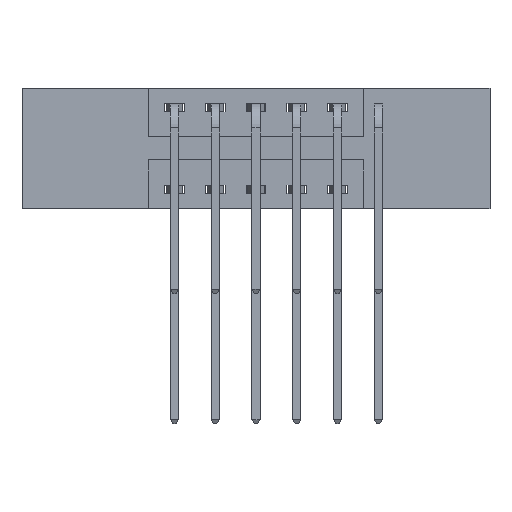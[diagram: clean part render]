
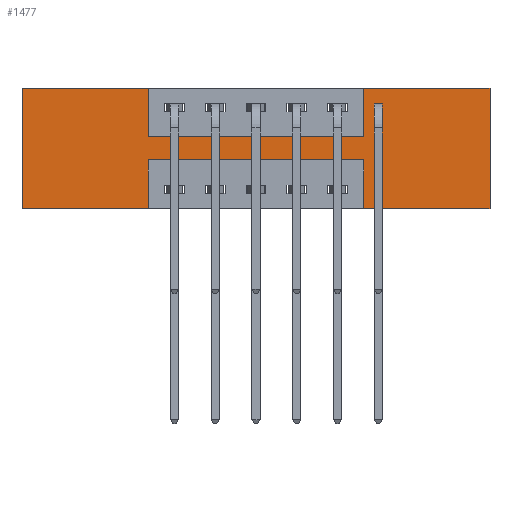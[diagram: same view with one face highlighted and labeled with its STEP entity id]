
A CAD part, front view. The second image highlights one B-rep face of the part: STEP entity #1477.
In plain terms, the highlighted planar face has unit normal (0, -1, 0).
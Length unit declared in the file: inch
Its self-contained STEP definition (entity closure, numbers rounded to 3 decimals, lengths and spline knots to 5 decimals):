
#90 = VERTEX_POINT ( 'NONE', #6516 ) ;
#178 = VERTEX_POINT ( 'NONE', #4496 ) ;
#186 = LINE ( 'NONE', #3003, #9487 ) ;
#317 = CARTESIAN_POINT ( 'NONE',  ( 1.0475, 0., -0.37 ) ) ;
#524 = ORIENTED_EDGE ( 'NONE', *, *, #1689, .F. ) ;
#607 = CARTESIAN_POINT ( 'NONE',  ( 0.3875, 0., 0. ) ) ;
#705 = VECTOR ( 'NONE', #9304, 39.37008 ) ;
#775 = LINE ( 'NONE', #5518, #5379 ) ;
#806 = DIRECTION ( 'NONE',  ( -1., 0., 0. ) ) ;
#931 = LINE ( 'NONE', #4889, #1242 ) ;
#1242 = VECTOR ( 'NONE', #5710, 39.37008 ) ;
#1294 = ORIENTED_EDGE ( 'NONE', *, *, #9307, .F. ) ;
#1436 = CARTESIAN_POINT ( 'NONE',  ( 0., 0., -0.37 ) ) ;
#1477 = ADVANCED_FACE ( 'NONE', ( #8497 ), #6266, .T. ) ;
#1542 = CARTESIAN_POINT ( 'NONE',  ( 1.435, 0., -0.37 ) ) ;
#1647 = DIRECTION ( 'NONE',  ( 0., -1., 0. ) ) ;
#1651 = DIRECTION ( 'NONE',  ( 0., 0., -1. ) ) ;
#1689 = EDGE_CURVE ( 'NONE', #90, #5949, #186, .T. ) ;
#1705 = ORIENTED_EDGE ( 'NONE', *, *, #2231, .F. ) ;
#1850 = EDGE_CURVE ( 'NONE', #178, #90, #4923, .T. ) ;
#2017 = VECTOR ( 'NONE', #806, 39.37008 ) ;
#2084 = VERTEX_POINT ( 'NONE', #607 ) ;
#2087 = ORIENTED_EDGE ( 'NONE', *, *, #7349, .F. ) ;
#2113 = EDGE_CURVE ( 'NONE', #6617, #7820, #9312, .T. ) ;
#2231 = EDGE_CURVE ( 'NONE', #5783, #5242, #9439, .T. ) ;
#2250 = DIRECTION ( 'NONE',  ( 0., 0., 1. ) ) ;
#2278 = DIRECTION ( 'NONE',  ( 1., 0., 0. ) ) ;
#2329 = CARTESIAN_POINT ( 'NONE',  ( 1.0475, 0., -0.22 ) ) ;
#2339 = LINE ( 'NONE', #8656, #8090 ) ;
#2481 = EDGE_CURVE ( 'NONE', #9753, #5783, #4009, .T. ) ;
#2495 = VECTOR ( 'NONE', #9743, 39.37008 ) ;
#2648 = LINE ( 'NONE', #8261, #2495 ) ;
#2877 = EDGE_LOOP ( 'NONE', ( #9728, #7736, #1705, #7483, #2087, #4880, #4223, #6678, #1294, #5826, #524, #3716 ) ) ;
#3003 = CARTESIAN_POINT ( 'NONE',  ( 0., 0., 0. ) ) ;
#3010 = EDGE_CURVE ( 'NONE', #7820, #6430, #2648, .T. ) ;
#3288 = AXIS2_PLACEMENT_3D ( 'NONE', #9418, #1647, #6869 ) ;
#3716 = ORIENTED_EDGE ( 'NONE', *, *, #1850, .F. ) ;
#3961 = VECTOR ( 'NONE', #6442, 39.37008 ) ;
#4009 = LINE ( 'NONE', #1436, #2017 ) ;
#4154 = VERTEX_POINT ( 'NONE', #6844 ) ;
#4171 = CARTESIAN_POINT ( 'NONE',  ( 0.3875, 0., -0.15 ) ) ;
#4223 = ORIENTED_EDGE ( 'NONE', *, *, #3010, .F. ) ;
#4496 = CARTESIAN_POINT ( 'NONE',  ( 0.3875, 0., -0.37 ) ) ;
#4744 = EDGE_CURVE ( 'NONE', #6430, #6102, #775, .T. ) ;
#4880 = ORIENTED_EDGE ( 'NONE', *, *, #4744, .F. ) ;
#4889 = CARTESIAN_POINT ( 'NONE',  ( 0.3875, 0., -0.37 ) ) ;
#4898 = DIRECTION ( 'NONE',  ( 1., 0., 0. ) ) ;
#4923 = LINE ( 'NONE', #6559, #8846 ) ;
#5032 = EDGE_CURVE ( 'NONE', #5949, #2084, #9067, .T. ) ;
#5114 = VECTOR ( 'NONE', #2278, 39.37008 ) ;
#5126 = VECTOR ( 'NONE', #10010, 39.37008 ) ;
#5242 = VERTEX_POINT ( 'NONE', #2329 ) ;
#5379 = VECTOR ( 'NONE', #4898, 39.37008 ) ;
#5499 = CARTESIAN_POINT ( 'NONE',  ( 1.0475, 0., -0.15 ) ) ;
#5518 = CARTESIAN_POINT ( 'NONE',  ( 0., 0., 0. ) ) ;
#5710 = DIRECTION ( 'NONE',  ( 0., 0., -1. ) ) ;
#5783 = VERTEX_POINT ( 'NONE', #317 ) ;
#5826 = ORIENTED_EDGE ( 'NONE', *, *, #5032, .F. ) ;
#5849 = DIRECTION ( 'NONE',  ( -1., 0., 0. ) ) ;
#5949 = VERTEX_POINT ( 'NONE', #8777 ) ;
#6102 = VERTEX_POINT ( 'NONE', #9581 ) ;
#6266 = PLANE ( 'NONE',  #3288 ) ;
#6278 = LINE ( 'NONE', #9433, #8589 ) ;
#6430 = VERTEX_POINT ( 'NONE', #6471 ) ;
#6442 = DIRECTION ( 'NONE',  ( 0., 0., 1. ) ) ;
#6471 = CARTESIAN_POINT ( 'NONE',  ( 1.0475, 0., 0. ) ) ;
#6516 = CARTESIAN_POINT ( 'NONE',  ( 0., 0., -0.37 ) ) ;
#6559 = CARTESIAN_POINT ( 'NONE',  ( 0., 0., -0.37 ) ) ;
#6617 = VERTEX_POINT ( 'NONE', #4171 ) ;
#6678 = ORIENTED_EDGE ( 'NONE', *, *, #2113, .F. ) ;
#6844 = CARTESIAN_POINT ( 'NONE',  ( 0.3875, 0., -0.22 ) ) ;
#6869 = DIRECTION ( 'NONE',  ( 0., 0., -1. ) ) ;
#6899 = LINE ( 'NONE', #8376, #705 ) ;
#6915 = CARTESIAN_POINT ( 'NONE',  ( 0., 0., 0. ) ) ;
#7349 = EDGE_CURVE ( 'NONE', #6102, #9753, #2339, .T. ) ;
#7483 = ORIENTED_EDGE ( 'NONE', *, *, #2481, .F. ) ;
#7736 = ORIENTED_EDGE ( 'NONE', *, *, #8236, .F. ) ;
#7820 = VERTEX_POINT ( 'NONE', #5499 ) ;
#7958 = CARTESIAN_POINT ( 'NONE',  ( 1.0475, 0., -0.37 ) ) ;
#8090 = VECTOR ( 'NONE', #1651, 39.37008 ) ;
#8236 = EDGE_CURVE ( 'NONE', #5242, #4154, #6899, .T. ) ;
#8261 = CARTESIAN_POINT ( 'NONE',  ( 1.0475, 0., 0. ) ) ;
#8376 = CARTESIAN_POINT ( 'NONE',  ( 0.3875, 0., -0.22 ) ) ;
#8497 = FACE_OUTER_BOUND ( 'NONE', #2877, .T. ) ;
#8589 = VECTOR ( 'NONE', #9386, 39.37008 ) ;
#8656 = CARTESIAN_POINT ( 'NONE',  ( 1.435, 0., 0. ) ) ;
#8777 = CARTESIAN_POINT ( 'NONE',  ( 0., 0., 0. ) ) ;
#8846 = VECTOR ( 'NONE', #5849, 39.37008 ) ;
#9067 = LINE ( 'NONE', #6915, #5126 ) ;
#9269 = CARTESIAN_POINT ( 'NONE',  ( 0.3875, 0., -0.15 ) ) ;
#9304 = DIRECTION ( 'NONE',  ( -1., 0., 0. ) ) ;
#9307 = EDGE_CURVE ( 'NONE', #2084, #6617, #6278, .T. ) ;
#9312 = LINE ( 'NONE', #9269, #5114 ) ;
#9386 = DIRECTION ( 'NONE',  ( 0., 0., -1. ) ) ;
#9418 = CARTESIAN_POINT ( 'NONE',  ( 0., 0., -0.37 ) ) ;
#9433 = CARTESIAN_POINT ( 'NONE',  ( 0.3875, 0., 0. ) ) ;
#9439 = LINE ( 'NONE', #7958, #3961 ) ;
#9487 = VECTOR ( 'NONE', #2250, 39.37008 ) ;
#9581 = CARTESIAN_POINT ( 'NONE',  ( 1.435, 0., 0. ) ) ;
#9728 = ORIENTED_EDGE ( 'NONE', *, *, #9846, .F. ) ;
#9743 = DIRECTION ( 'NONE',  ( 0., 0., 1. ) ) ;
#9753 = VERTEX_POINT ( 'NONE', #1542 ) ;
#9846 = EDGE_CURVE ( 'NONE', #4154, #178, #931, .T. ) ;
#10010 = DIRECTION ( 'NONE',  ( 1., 0., 0. ) ) ;
